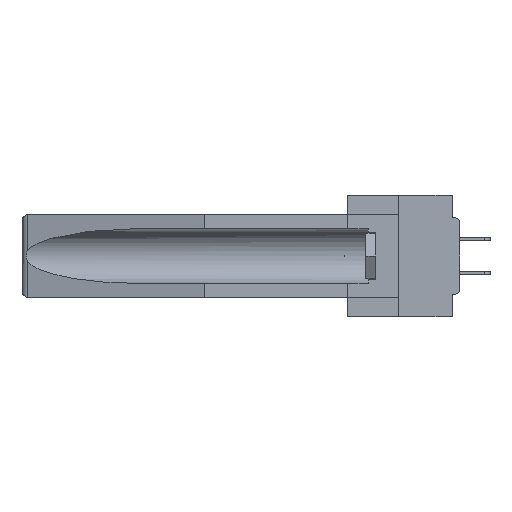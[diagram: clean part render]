
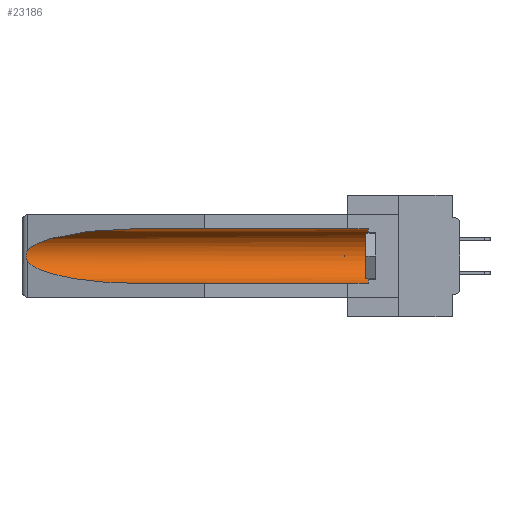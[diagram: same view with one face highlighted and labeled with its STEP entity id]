
A CAD part, left-side view. The second image highlights one B-rep face of the part: STEP entity #23186.
In plain terms, the highlighted cylindrical face has radius 2.857 mm (diameter 5.715 mm), a partial arc.
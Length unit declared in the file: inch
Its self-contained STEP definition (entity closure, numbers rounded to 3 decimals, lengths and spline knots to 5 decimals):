
#241 = DIRECTION ( 'NONE',  ( 0., -1., 0. ) ) ;
#643 = CARTESIAN_POINT ( 'NONE',  ( 0.155, 1.07973, -0.284 ) ) ;
#2196 = DIRECTION ( 'NONE',  ( 0., 1., 0. ) ) ;
#2343 = VERTEX_POINT ( 'NONE', #45268 ) ;
#3247 = EDGE_CURVE ( 'NONE', #12859, #38367, #22493, .T. ) ;
#3499 = LINE ( 'NONE', #20931, #16813 ) ;
#4190 = CARTESIAN_POINT ( 'NONE',  ( 0.26537, 1.52718, -0.19328 ) ) ;
#4263 = DIRECTION ( 'NONE',  ( 0., 0., 1. ) ) ;
#4453 = CARTESIAN_POINT ( 'NONE',  ( 0.155, 0.126, -0.059 ) ) ;
#5909 = CARTESIAN_POINT ( 'NONE',  ( 0.155, -0.30754, -0.1715 ) ) ;
#6380 = FACE_OUTER_BOUND ( 'NONE', #23772, .T. ) ;
#7939 = EDGE_CURVE ( 'NONE', #38367, #2343, #39670, .T. ) ;
#10876 = CARTESIAN_POINT ( 'NONE',  ( 0.155, 0.126, -0.1715 ) ) ;
#11029 = CARTESIAN_POINT ( 'NONE',  ( 0.155, 0.126, -0.284 ) ) ;
#11631 = EDGE_CURVE ( 'NONE', #35707, #12859, #34930, .T. ) ;
#12859 = VERTEX_POINT ( 'NONE', #47431 ) ;
#12864 = DIRECTION ( 'NONE',  ( 0., 0., 1. ) ) ;
#13342 = CARTESIAN_POINT ( 'NONE',  ( 0.155, 1.07973, -0.059 ) ) ;
#13523 = AXIS2_PLACEMENT_3D ( 'NONE', #10876, #241, #4263 ) ;
#16624 = CIRCLE ( 'NONE', #13523, 0.1125 ) ;
#16813 = VECTOR ( 'NONE', #39653, 39.37008 ) ;
#16916 = CARTESIAN_POINT ( 'NONE',  ( 0.2673, 1.5327, -0.16383 ) ) ;
#18751 = CARTESIAN_POINT ( 'NONE',  ( 0.155, -0.30754, -0.059 ) ) ;
#18967 = ORIENTED_EDGE ( 'NONE', *, *, #22899, .F. ) ;
#20495 = VECTOR ( 'NONE', #37461, 39.37008 ) ;
#20745 = CARTESIAN_POINT ( 'NONE',  ( 0.2675, 1.53308, -0.16763 ) ) ;
#20931 = CARTESIAN_POINT ( 'NONE',  ( 0.155, -0.30754, -0.284 ) ) ;
#22493 =( BOUNDED_CURVE ( )  B_SPLINE_CURVE ( 3, ( #13342, #28081, #39099, #38478 ),
 .UNSPECIFIED., .F., .F. ) 
 B_SPLINE_CURVE_WITH_KNOTS ( ( 4, 4 ),
 ( 4.71239, 6.08839 ),
 .UNSPECIFIED. ) 
 CURVE ( )  GEOMETRIC_REPRESENTATION_ITEM ( )  RATIONAL_B_SPLINE_CURVE ( ( 1., 0.848, 0.848, 1. ) ) 
 REPRESENTATION_ITEM ( '' )  );
#22899 = EDGE_CURVE ( 'NONE', #30433, #43999, #3499, .T. ) ;
#23186 = ADVANCED_FACE ( 'NONE', ( #6380 ), #32312, .F. ) ;
#23653 = CARTESIAN_POINT ( 'NONE',  ( 0.2675, 1.53308, -0.17534 ) ) ;
#23772 = EDGE_LOOP ( 'NONE', ( #39444, #29301, #35064, #18967, #36537, #36525 ) ) ;
#23801 = CARTESIAN_POINT ( 'NONE',  ( 0.26537, 1.52718, -0.19328 ) ) ;
#27341 = CARTESIAN_POINT ( 'NONE',  ( 0.2673, 1.53269, -0.17917 ) ) ;
#27926 = CARTESIAN_POINT ( 'NONE',  ( 0.26537, 1.52718, -0.14972 ) ) ;
#28081 = CARTESIAN_POINT ( 'NONE',  ( 0.21114, 1.30732, -0.059 ) ) ;
#29301 = ORIENTED_EDGE ( 'NONE', *, *, #7939, .T. ) ;
#30433 = VERTEX_POINT ( 'NONE', #11029 ) ;
#30550 = EDGE_CURVE ( 'NONE', #30433, #35707, #16624, .T. ) ;
#31058 = CARTESIAN_POINT ( 'NONE',  ( 0.26655, 1.53094, -0.18657 ) ) ;
#32312 = CYLINDRICAL_SURFACE ( 'NONE', #40827, 0.1125 ) ;
#33706 = CARTESIAN_POINT ( 'NONE',  ( 0.21114, 1.30732, -0.284 ) ) ;
#34029 =( BOUNDED_CURVE ( )  B_SPLINE_CURVE ( 3, ( #4190, #40939, #33706, #643 ),
 .UNSPECIFIED., .F., .F. ) 
 B_SPLINE_CURVE_WITH_KNOTS ( ( 4, 4 ),
 ( 0.1948, 1.5708 ),
 .UNSPECIFIED. ) 
 CURVE ( )  GEOMETRIC_REPRESENTATION_ITEM ( )  RATIONAL_B_SPLINE_CURVE ( ( 1., 0.848, 0.848, 1. ) ) 
 REPRESENTATION_ITEM ( '' )  );
#34930 = LINE ( 'NONE', #18751, #20495 ) ;
#35064 = ORIENTED_EDGE ( 'NONE', *, *, #46038, .T. ) ;
#35271 = CARTESIAN_POINT ( 'NONE',  ( 0.26654, 1.53092, -0.15636 ) ) ;
#35707 = VERTEX_POINT ( 'NONE', #4453 ) ;
#36525 = ORIENTED_EDGE ( 'NONE', *, *, #11631, .T. ) ;
#36537 = ORIENTED_EDGE ( 'NONE', *, *, #30550, .T. ) ;
#37461 = DIRECTION ( 'NONE',  ( 0., 1., 0. ) ) ;
#38367 = VERTEX_POINT ( 'NONE', #27926 ) ;
#38478 = CARTESIAN_POINT ( 'NONE',  ( 0.26537, 1.52718, -0.14972 ) ) ;
#38687 = CARTESIAN_POINT ( 'NONE',  ( 0.26537, 1.52718, -0.14972 ) ) ;
#39099 = CARTESIAN_POINT ( 'NONE',  ( 0.25451, 1.48313, -0.09465 ) ) ;
#39444 = ORIENTED_EDGE ( 'NONE', *, *, #3247, .T. ) ;
#39653 = DIRECTION ( 'NONE',  ( 0., 1., 0. ) ) ;
#39670 = B_SPLINE_CURVE_WITH_KNOTS ( 'NONE', 3,
 ( #38687, #42327, #35271, #16916, #20745, #23653, #27341, #31058, #46071, #23801 ),
 .UNSPECIFIED., .F., .F.,
 ( 4, 2, 2, 2, 4 ),
 ( 0., 0.00029, 0.00058, 0.00087, 0.00117 ),
 .UNSPECIFIED. ) ;
#40827 = AXIS2_PLACEMENT_3D ( 'NONE', #5909, #2196, #12864 ) ;
#40939 = CARTESIAN_POINT ( 'NONE',  ( 0.25451, 1.48313, -0.24835 ) ) ;
#42322 = CARTESIAN_POINT ( 'NONE',  ( 0.155, 1.07973, -0.284 ) ) ;
#42327 = CARTESIAN_POINT ( 'NONE',  ( 0.26597, 1.52961, -0.15275 ) ) ;
#43999 = VERTEX_POINT ( 'NONE', #42322 ) ;
#45268 = CARTESIAN_POINT ( 'NONE',  ( 0.26537, 1.52718, -0.19328 ) ) ;
#46038 = EDGE_CURVE ( 'NONE', #2343, #43999, #34029, .T. ) ;
#46071 = CARTESIAN_POINT ( 'NONE',  ( 0.26597, 1.5296, -0.19026 ) ) ;
#47431 = CARTESIAN_POINT ( 'NONE',  ( 0.155, 1.07973, -0.059 ) ) ;
